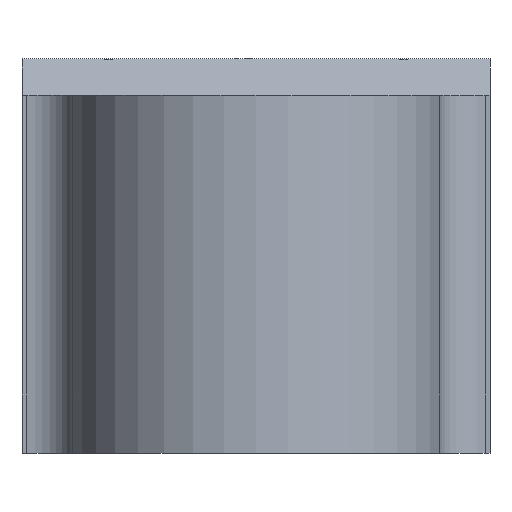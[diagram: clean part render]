
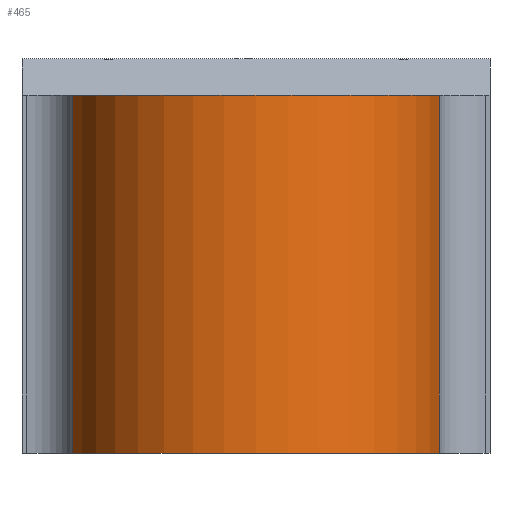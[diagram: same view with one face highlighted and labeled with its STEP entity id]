
A CAD part, front view. The second image highlights one B-rep face of the part: STEP entity #465.
In plain terms, the highlighted cylindrical face has radius 12.7 mm (diameter 25.4 mm), a partial arc.
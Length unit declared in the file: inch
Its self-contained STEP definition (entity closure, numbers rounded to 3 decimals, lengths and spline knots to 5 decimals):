
#52=FACE_OUTER_BOUND('',#77,.T.);
#77=EDGE_LOOP('',(#330,#331,#332,#333));
#110=LINE('',#698,#156);
#112=LINE('',#706,#158);
#156=VECTOR('',#560,0.3937);
#158=VECTOR('',#568,0.3937);
#204=CIRCLE('',#513,0.5);
#205=CIRCLE('',#514,0.5);
#215=VERTEX_POINT('',#695);
#216=VERTEX_POINT('',#697);
#218=VERTEX_POINT('',#703);
#219=VERTEX_POINT('',#705);
#261=EDGE_CURVE('',#215,#216,#110,.T.);
#264=EDGE_CURVE('',#215,#218,#204,.T.);
#265=EDGE_CURVE('',#219,#218,#112,.T.);
#266=EDGE_CURVE('',#216,#219,#205,.T.);
#330=ORIENTED_EDGE('',*,*,#261,.F.);
#331=ORIENTED_EDGE('',*,*,#264,.T.);
#332=ORIENTED_EDGE('',*,*,#265,.F.);
#333=ORIENTED_EDGE('',*,*,#266,.F.);
#459=CYLINDRICAL_SURFACE('',#512,0.5);
#465=ADVANCED_FACE('',(#52),#459,.T.);
#512=AXIS2_PLACEMENT_3D('',#702,#564,#565);
#513=AXIS2_PLACEMENT_3D('',#704,#566,#567);
#514=AXIS2_PLACEMENT_3D('',#707,#569,#570);
#560=DIRECTION('',(0.,0.,-1.));
#564=DIRECTION('center_axis',(0.,0.,1.));
#565=DIRECTION('ref_axis',(1.,0.,0.));
#566=DIRECTION('center_axis',(0.,0.,-1.));
#567=DIRECTION('ref_axis',(1.,0.,0.));
#568=DIRECTION('',(0.,0.,1.));
#569=DIRECTION('center_axis',(0.,0.,-1.));
#570=DIRECTION('ref_axis',(1.,0.,0.));
#695=CARTESIAN_POINT('',(1.1149,-0.35,0.3305));
#697=CARTESIAN_POINT('',(1.1149,-0.35,-0.625));
#698=CARTESIAN_POINT('',(1.1149,-0.35,-0.625));
#702=CARTESIAN_POINT('Origin',(0.625,-0.25,-0.625));
#703=CARTESIAN_POINT('',(0.1351,-0.35,0.3305));
#704=CARTESIAN_POINT('Origin',(0.625,-0.25,0.3305));
#705=CARTESIAN_POINT('',(0.1351,-0.35,-0.625));
#706=CARTESIAN_POINT('',(0.1351,-0.35,-0.625));
#707=CARTESIAN_POINT('Origin',(0.625,-0.25,-0.625));
